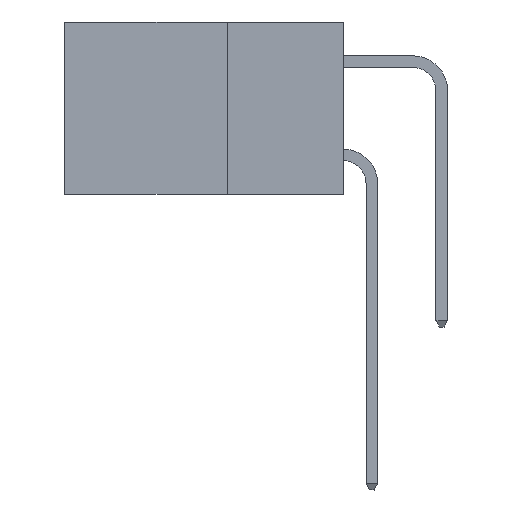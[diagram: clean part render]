
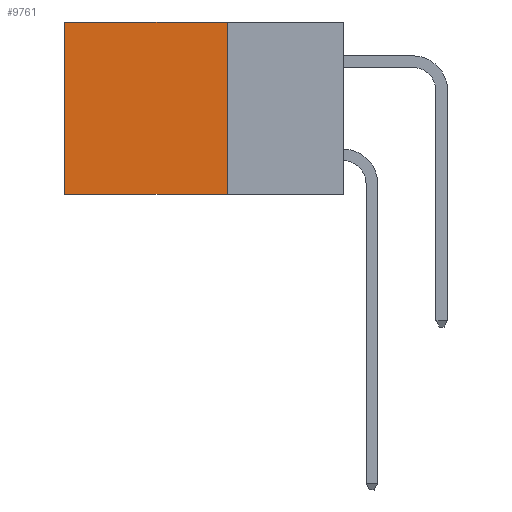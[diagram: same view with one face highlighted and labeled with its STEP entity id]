
A CAD part, left-side view. The second image highlights one B-rep face of the part: STEP entity #9761.
In plain terms, the highlighted planar face has unit normal (-1, 0, 0).
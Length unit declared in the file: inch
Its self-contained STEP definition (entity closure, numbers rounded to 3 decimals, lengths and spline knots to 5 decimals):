
#1040 = CARTESIAN_POINT ( 'NONE',  ( 0.2615, 0.25, 0. ) ) ;
#1964 = VECTOR ( 'NONE', #3682, 39.37008 ) ;
#2382 = LINE ( 'NONE', #8913, #9419 ) ;
#2693 = VECTOR ( 'NONE', #7136, 39.37008 ) ;
#2938 = LINE ( 'NONE', #10282, #2693 ) ;
#3682 = DIRECTION ( 'NONE',  ( 0., 1., 0. ) ) ;
#4266 = PLANE ( 'NONE',  #7025 ) ;
#4326 = DIRECTION ( 'NONE',  ( 0., 0., -1. ) ) ;
#4702 = EDGE_CURVE ( 'NONE', #7080, #6075, #2938, .T. ) ;
#4989 = CARTESIAN_POINT ( 'NONE',  ( 0.2615, 0.6, -0.37 ) ) ;
#5227 = DIRECTION ( 'NONE',  ( 0., 1., 0. ) ) ;
#5377 = CARTESIAN_POINT ( 'NONE',  ( 0.2615, 0.25, -0.37 ) ) ;
#6006 = EDGE_CURVE ( 'NONE', #11769, #11159, #2382, .T. ) ;
#6075 = VERTEX_POINT ( 'NONE', #4989 ) ;
#6976 = ORIENTED_EDGE ( 'NONE', *, *, #6006, .F. ) ;
#7025 = AXIS2_PLACEMENT_3D ( 'NONE', #5377, #12849, #4326 ) ;
#7080 = VERTEX_POINT ( 'NONE', #12706 ) ;
#7136 = DIRECTION ( 'NONE',  ( 0., 0., -1. ) ) ;
#7703 = VECTOR ( 'NONE', #5227, 39.37008 ) ;
#7879 = DIRECTION ( 'NONE',  ( 0., 0., -1. ) ) ;
#8133 = CARTESIAN_POINT ( 'NONE',  ( 0.2615, 0.25, -0.37 ) ) ;
#8266 = LINE ( 'NONE', #8133, #1964 ) ;
#8913 = CARTESIAN_POINT ( 'NONE',  ( 0.2615, 0.25, -0.37 ) ) ;
#9165 = ORIENTED_EDGE ( 'NONE', *, *, #4702, .T. ) ;
#9353 = CARTESIAN_POINT ( 'NONE',  ( 0.2615, 0.25, 0. ) ) ;
#9419 = VECTOR ( 'NONE', #7879, 39.37008 ) ;
#9558 = LINE ( 'NONE', #9353, #7703 ) ;
#9570 = EDGE_LOOP ( 'NONE', ( #9165, #13449, #6976, #13507 ) ) ;
#9613 = EDGE_CURVE ( 'NONE', #11159, #6075, #8266, .T. ) ;
#9761 = ADVANCED_FACE ( 'NONE', ( #10528 ), #4266, .F. ) ;
#10282 = CARTESIAN_POINT ( 'NONE',  ( 0.2615, 0.6, -0.37 ) ) ;
#10528 = FACE_OUTER_BOUND ( 'NONE', #9570, .T. ) ;
#10830 = EDGE_CURVE ( 'NONE', #11769, #7080, #9558, .T. ) ;
#11159 = VERTEX_POINT ( 'NONE', #12869 ) ;
#11769 = VERTEX_POINT ( 'NONE', #1040 ) ;
#12706 = CARTESIAN_POINT ( 'NONE',  ( 0.2615, 0.6, 0. ) ) ;
#12849 = DIRECTION ( 'NONE',  ( 1., 0., 0. ) ) ;
#12869 = CARTESIAN_POINT ( 'NONE',  ( 0.2615, 0.25, -0.37 ) ) ;
#13449 = ORIENTED_EDGE ( 'NONE', *, *, #9613, .F. ) ;
#13507 = ORIENTED_EDGE ( 'NONE', *, *, #10830, .T. ) ;
